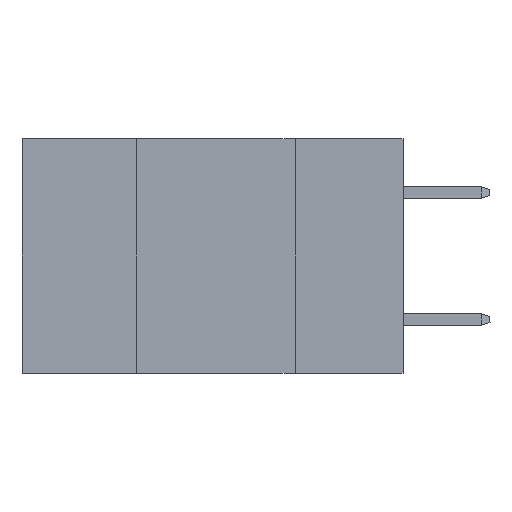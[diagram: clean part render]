
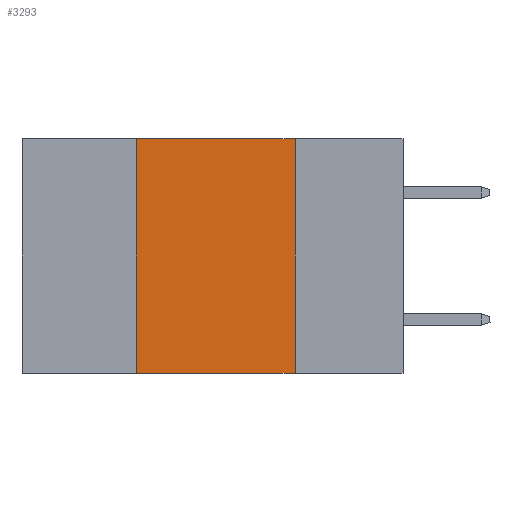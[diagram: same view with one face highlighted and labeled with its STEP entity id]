
A CAD part, left-side view. The second image highlights one B-rep face of the part: STEP entity #3293.
In plain terms, the highlighted planar face has unit normal (-1, 0, 0).
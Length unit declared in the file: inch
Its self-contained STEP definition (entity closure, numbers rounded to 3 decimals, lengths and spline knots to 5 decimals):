
#807 = FACE_OUTER_BOUND ( 'NONE', #8276, .T. ) ;
#1744 = EDGE_CURVE ( 'NONE', #10709, #9662, #3769, .T. ) ;
#2072 = DIRECTION ( 'NONE',  ( 1., 0., 0. ) ) ;
#2147 = PLANE ( 'NONE',  #13943 ) ;
#2199 = DIRECTION ( 'NONE',  ( 0., -1., 0. ) ) ;
#2219 = VECTOR ( 'NONE', #2818, 39.37008 ) ;
#2344 = CARTESIAN_POINT ( 'NONE',  ( 0., 0.6, 0. ) ) ;
#2818 = DIRECTION ( 'NONE',  ( 0., -1., 0. ) ) ;
#3157 = LINE ( 'NONE', #7976, #13076 ) ;
#3293 = ADVANCED_FACE ( 'NONE', ( #807 ), #2147, .F. ) ;
#3769 = LINE ( 'NONE', #8367, #4301 ) ;
#3953 = CARTESIAN_POINT ( 'NONE',  ( 0., 0.17, -0.37 ) ) ;
#4038 = LINE ( 'NONE', #12292, #2219 ) ;
#4288 = CARTESIAN_POINT ( 'NONE',  ( 0., 0.6, 0. ) ) ;
#4301 = VECTOR ( 'NONE', #7070, 39.37008 ) ;
#4573 = ORIENTED_EDGE ( 'NONE', *, *, #9491, .F. ) ;
#7070 = DIRECTION ( 'NONE',  ( 0., 0., 1. ) ) ;
#7491 = VERTEX_POINT ( 'NONE', #3953 ) ;
#7619 = ORIENTED_EDGE ( 'NONE', *, *, #12333, .F. ) ;
#7976 = CARTESIAN_POINT ( 'NONE',  ( 0., 0.17, 0. ) ) ;
#8276 = EDGE_LOOP ( 'NONE', ( #4573, #7619, #9158, #12575 ) ) ;
#8367 = CARTESIAN_POINT ( 'NONE',  ( 0., 0.42, 0. ) ) ;
#8510 = VECTOR ( 'NONE', #2199, 39.37008 ) ;
#9158 = ORIENTED_EDGE ( 'NONE', *, *, #1744, .F. ) ;
#9491 = EDGE_CURVE ( 'NONE', #14608, #7491, #3157, .T. ) ;
#9662 = VERTEX_POINT ( 'NONE', #10440 ) ;
#9667 = CARTESIAN_POINT ( 'NONE',  ( 0., 0.42, -0.37 ) ) ;
#10440 = CARTESIAN_POINT ( 'NONE',  ( 0., 0.42, 0. ) ) ;
#10709 = VERTEX_POINT ( 'NONE', #9667 ) ;
#12262 = DIRECTION ( 'NONE',  ( 0., 0., -1. ) ) ;
#12292 = CARTESIAN_POINT ( 'NONE',  ( 0., 0.6, -0.37 ) ) ;
#12333 = EDGE_CURVE ( 'NONE', #9662, #14608, #14724, .T. ) ;
#12575 = ORIENTED_EDGE ( 'NONE', *, *, #12660, .T. ) ;
#12660 = EDGE_CURVE ( 'NONE', #10709, #7491, #4038, .T. ) ;
#13076 = VECTOR ( 'NONE', #12262, 39.37008 ) ;
#13943 = AXIS2_PLACEMENT_3D ( 'NONE', #4288, #2072, #14741 ) ;
#14608 = VERTEX_POINT ( 'NONE', #14767 ) ;
#14724 = LINE ( 'NONE', #2344, #8510 ) ;
#14741 = DIRECTION ( 'NONE',  ( 0., 0., -1. ) ) ;
#14767 = CARTESIAN_POINT ( 'NONE',  ( 0., 0.17, 0. ) ) ;
